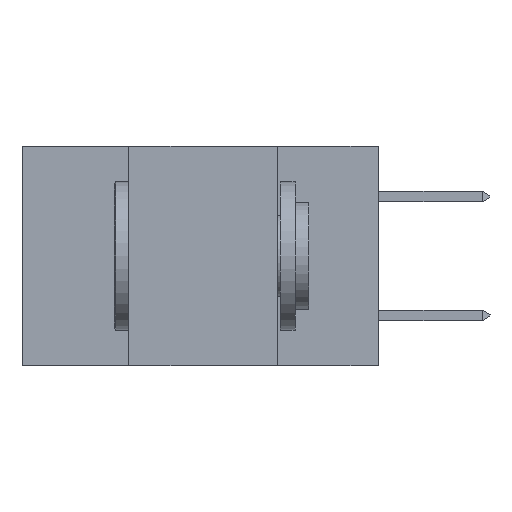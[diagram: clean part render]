
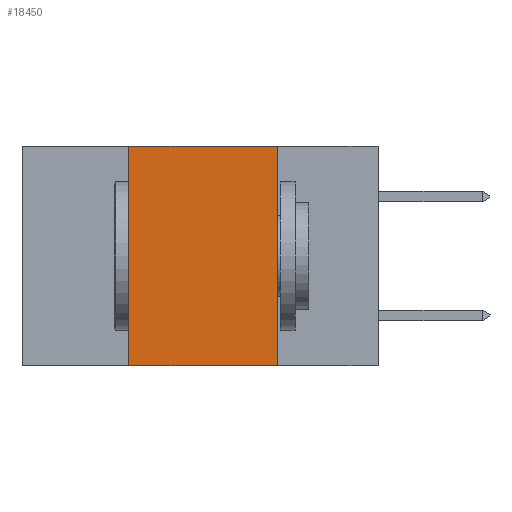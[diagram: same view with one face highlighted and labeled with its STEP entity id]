
A CAD part, left-side view. The second image highlights one B-rep face of the part: STEP entity #18450.
In plain terms, the highlighted planar face has unit normal (-1, 0, 0).
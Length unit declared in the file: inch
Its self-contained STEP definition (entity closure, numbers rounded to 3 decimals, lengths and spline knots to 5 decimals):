
#753 = ORIENTED_EDGE ( 'NONE', *, *, #11947, .F. ) ;
#1083 = CARTESIAN_POINT ( 'NONE',  ( 0., 0.6, 0. ) ) ;
#1352 = ORIENTED_EDGE ( 'NONE', *, *, #6910, .F. ) ;
#2945 = PLANE ( 'NONE',  #20381 ) ;
#3677 = EDGE_LOOP ( 'NONE', ( #1352, #10758, #753, #4592 ) ) ;
#4592 = ORIENTED_EDGE ( 'NONE', *, *, #10675, .T. ) ;
#4838 = CARTESIAN_POINT ( 'NONE',  ( 0., 0.6, 0. ) ) ;
#5380 = LINE ( 'NONE', #19282, #10360 ) ;
#6348 = DIRECTION ( 'NONE',  ( 0., 0., -1. ) ) ;
#6731 = DIRECTION ( 'NONE',  ( 1., 0., 0. ) ) ;
#6910 = EDGE_CURVE ( 'NONE', #16184, #16183, #17846, .T. ) ;
#7153 = CARTESIAN_POINT ( 'NONE',  ( 0., 0.42, -0.37 ) ) ;
#7188 = CARTESIAN_POINT ( 'NONE',  ( 0., 0.17, -0.37 ) ) ;
#7224 = VECTOR ( 'NONE', #6348, 39.37008 ) ;
#8077 = VERTEX_POINT ( 'NONE', #10053 ) ;
#10053 = CARTESIAN_POINT ( 'NONE',  ( 0., 0.42, -0.37 ) ) ;
#10360 = VECTOR ( 'NONE', #15496, 39.37008 ) ;
#10532 = VECTOR ( 'NONE', #14278, 39.37008 ) ;
#10675 = EDGE_CURVE ( 'NONE', #8077, #16183, #5380, .T. ) ;
#10758 = ORIENTED_EDGE ( 'NONE', *, *, #13234, .F. ) ;
#11947 = EDGE_CURVE ( 'NONE', #8077, #22543, #14461, .T. ) ;
#13234 = EDGE_CURVE ( 'NONE', #22543, #16184, #22314, .T. ) ;
#14278 = DIRECTION ( 'NONE',  ( 0., -1., 0. ) ) ;
#14461 = LINE ( 'NONE', #7153, #23845 ) ;
#14661 = DIRECTION ( 'NONE',  ( 0., 0., 1. ) ) ;
#15496 = DIRECTION ( 'NONE',  ( 0., -1., 0. ) ) ;
#16183 = VERTEX_POINT ( 'NONE', #7188 ) ;
#16184 = VERTEX_POINT ( 'NONE', #20378 ) ;
#17846 = LINE ( 'NONE', #19544, #7224 ) ;
#18450 = ADVANCED_FACE ( 'NONE', ( #23812 ), #2945, .F. ) ;
#19282 = CARTESIAN_POINT ( 'NONE',  ( 0., 0.6, -0.37 ) ) ;
#19544 = CARTESIAN_POINT ( 'NONE',  ( 0., 0.17, -0.37 ) ) ;
#19910 = DIRECTION ( 'NONE',  ( 0., 0., -1. ) ) ;
#20378 = CARTESIAN_POINT ( 'NONE',  ( 0., 0.17, 0. ) ) ;
#20381 = AXIS2_PLACEMENT_3D ( 'NONE', #4838, #6731, #19910 ) ;
#21651 = CARTESIAN_POINT ( 'NONE',  ( 0., 0.42, 0. ) ) ;
#22314 = LINE ( 'NONE', #1083, #10532 ) ;
#22543 = VERTEX_POINT ( 'NONE', #21651 ) ;
#23812 = FACE_OUTER_BOUND ( 'NONE', #3677, .T. ) ;
#23845 = VECTOR ( 'NONE', #14661, 39.37008 ) ;
